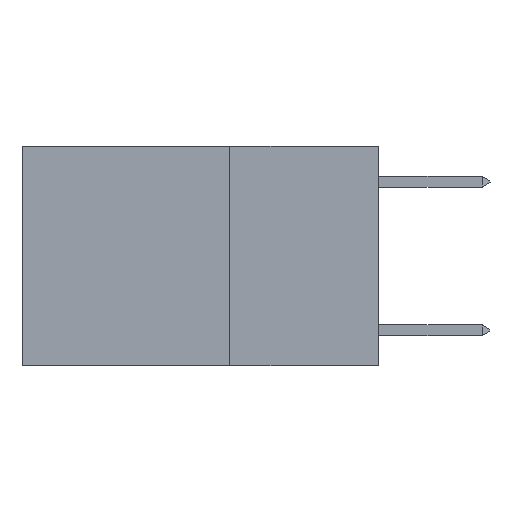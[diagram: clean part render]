
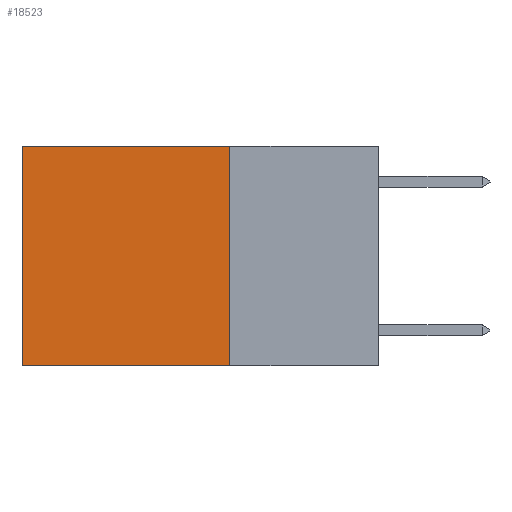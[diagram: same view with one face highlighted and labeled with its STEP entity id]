
A CAD part, left-side view. The second image highlights one B-rep face of the part: STEP entity #18523.
In plain terms, the highlighted planar face has unit normal (-1, 0, 0).
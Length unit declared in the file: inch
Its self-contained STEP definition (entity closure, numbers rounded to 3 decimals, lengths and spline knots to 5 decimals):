
#1615 = PLANE ( 'NONE',  #20272 ) ;
#1818 = VERTEX_POINT ( 'NONE', #14243 ) ;
#2678 = CARTESIAN_POINT ( 'NONE',  ( 0.2625, 0.25, 0. ) ) ;
#3668 = DIRECTION ( 'NONE',  ( 0., 0., -1. ) ) ;
#3934 = EDGE_CURVE ( 'NONE', #7274, #17779, #7270, .T. ) ;
#4022 = LINE ( 'NONE', #5957, #8197 ) ;
#4163 = CARTESIAN_POINT ( 'NONE',  ( 0.2625, 0.6, 0. ) ) ;
#4172 = VERTEX_POINT ( 'NONE', #10759 ) ;
#4242 = DIRECTION ( 'NONE',  ( 0., 0., -1. ) ) ;
#5854 = LINE ( 'NONE', #19676, #14782 ) ;
#5957 = CARTESIAN_POINT ( 'NONE',  ( 0.2625, 0.6, 0. ) ) ;
#5976 = ORIENTED_EDGE ( 'NONE', *, *, #3934, .T. ) ;
#6644 = ORIENTED_EDGE ( 'NONE', *, *, #16751, .T. ) ;
#7070 = FACE_OUTER_BOUND ( 'NONE', #22103, .T. ) ;
#7270 = LINE ( 'NONE', #2678, #11646 ) ;
#7274 = VERTEX_POINT ( 'NONE', #15929 ) ;
#7621 = CARTESIAN_POINT ( 'NONE',  ( 0.2625, 0.25, -0.37 ) ) ;
#8197 = VECTOR ( 'NONE', #4242, 39.37008 ) ;
#9246 = ORIENTED_EDGE ( 'NONE', *, *, #18114, .F. ) ;
#10759 = CARTESIAN_POINT ( 'NONE',  ( 0.2625, 0.25, -0.37 ) ) ;
#11281 = LINE ( 'NONE', #7621, #16005 ) ;
#11646 = VECTOR ( 'NONE', #14250, 39.37008 ) ;
#12342 = CARTESIAN_POINT ( 'NONE',  ( 0.2625, 0.25, 0. ) ) ;
#14243 = CARTESIAN_POINT ( 'NONE',  ( 0.2625, 0.6, -0.37 ) ) ;
#14250 = DIRECTION ( 'NONE',  ( 0., 1., 0. ) ) ;
#14782 = VECTOR ( 'NONE', #18181, 39.37008 ) ;
#15918 = ORIENTED_EDGE ( 'NONE', *, *, #21819, .F. ) ;
#15929 = CARTESIAN_POINT ( 'NONE',  ( 0.2625, 0.25, 0. ) ) ;
#16005 = VECTOR ( 'NONE', #16644, 39.37008 ) ;
#16644 = DIRECTION ( 'NONE',  ( 0., 1., 0. ) ) ;
#16751 = EDGE_CURVE ( 'NONE', #17779, #1818, #4022, .T. ) ;
#17779 = VERTEX_POINT ( 'NONE', #4163 ) ;
#18114 = EDGE_CURVE ( 'NONE', #7274, #4172, #5854, .T. ) ;
#18181 = DIRECTION ( 'NONE',  ( 0., 0., -1. ) ) ;
#18523 = ADVANCED_FACE ( 'NONE', ( #7070 ), #1615, .F. ) ;
#19308 = DIRECTION ( 'NONE',  ( 1., 0., 0. ) ) ;
#19676 = CARTESIAN_POINT ( 'NONE',  ( 0.2625, 0.25, 0. ) ) ;
#20272 = AXIS2_PLACEMENT_3D ( 'NONE', #12342, #19308, #3668 ) ;
#21819 = EDGE_CURVE ( 'NONE', #4172, #1818, #11281, .T. ) ;
#22103 = EDGE_LOOP ( 'NONE', ( #6644, #15918, #9246, #5976 ) ) ;
